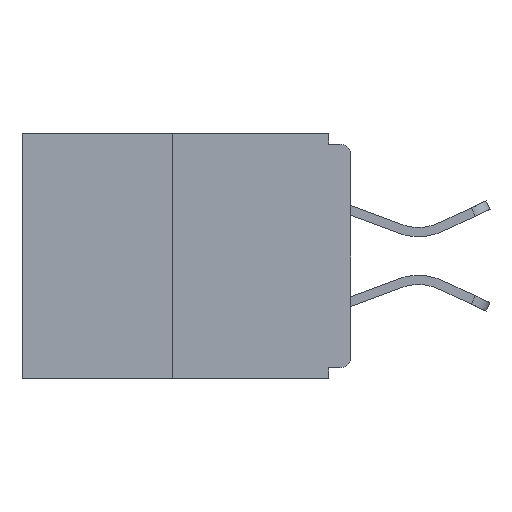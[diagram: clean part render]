
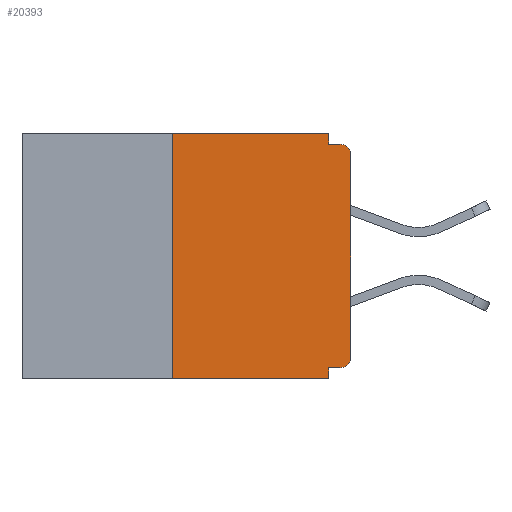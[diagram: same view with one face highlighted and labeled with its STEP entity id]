
A CAD part, left-side view. The second image highlights one B-rep face of the part: STEP entity #20393.
In plain terms, the highlighted planar face has unit normal (-1, 0, 0).
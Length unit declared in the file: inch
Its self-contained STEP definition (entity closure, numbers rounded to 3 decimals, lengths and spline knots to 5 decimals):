
#811 = DIRECTION ( 'NONE',  ( 0., -1., 0. ) ) ;
#1473 = CARTESIAN_POINT ( 'NONE',  ( 0., 0.031, 0. ) ) ;
#1618 = VECTOR ( 'NONE', #811, 39.37008 ) ;
#1887 = VERTEX_POINT ( 'NONE', #28854 ) ;
#2306 = CARTESIAN_POINT ( 'NONE',  ( 0., 0.015, -0.015 ) ) ;
#2321 = VERTEX_POINT ( 'NONE', #1473 ) ;
#2989 = DIRECTION ( 'NONE',  ( 1., 0., 0. ) ) ;
#3128 = CARTESIAN_POINT ( 'NONE',  ( 0., 0.015, -0.328 ) ) ;
#3155 = DIRECTION ( 'NONE',  ( 0., -1., 0. ) ) ;
#3368 = LINE ( 'NONE', #21479, #1618 ) ;
#3377 = VERTEX_POINT ( 'NONE', #6656 ) ;
#3804 = CARTESIAN_POINT ( 'NONE',  ( 0., 0.25, 0. ) ) ;
#4388 = AXIS2_PLACEMENT_3D ( 'NONE', #17617, #29236, #29541 ) ;
#4418 = CARTESIAN_POINT ( 'NONE',  ( 0., 0., -0.313 ) ) ;
#4719 = ORIENTED_EDGE ( 'NONE', *, *, #23878, .F. ) ;
#4732 = VERTEX_POINT ( 'NONE', #3804 ) ;
#4808 = VECTOR ( 'NONE', #23315, 39.37008 ) ;
#5930 = VERTEX_POINT ( 'NONE', #7351 ) ;
#6019 = LINE ( 'NONE', #22008, #26554 ) ;
#6042 = ORIENTED_EDGE ( 'NONE', *, *, #11639, .F. ) ;
#6083 = CARTESIAN_POINT ( 'NONE',  ( 0., 0.031, 0. ) ) ;
#6374 = LINE ( 'NONE', #18257, #24286 ) ;
#6656 = CARTESIAN_POINT ( 'NONE',  ( 0., 0.031, -0.015 ) ) ;
#7351 = CARTESIAN_POINT ( 'NONE',  ( 0., 0.031, -0.328 ) ) ;
#8089 = PLANE ( 'NONE',  #16899 ) ;
#9112 = EDGE_CURVE ( 'NONE', #13773, #11998, #25568, .T. ) ;
#9196 = CARTESIAN_POINT ( 'NONE',  ( 0., 0., -0.328 ) ) ;
#10501 = EDGE_CURVE ( 'NONE', #18077, #13773, #27045, .T. ) ;
#11170 = EDGE_LOOP ( 'NONE', ( #15086, #4719, #16507, #25999, #6042, #23730, #26352, #15635, #24366, #24740 ) ) ;
#11278 = CARTESIAN_POINT ( 'NONE',  ( 0., 0.015, -0.03 ) ) ;
#11639 = EDGE_CURVE ( 'NONE', #18077, #5930, #27781, .T. ) ;
#11921 = DIRECTION ( 'NONE',  ( 0., 1., 0. ) ) ;
#11998 = VERTEX_POINT ( 'NONE', #24683 ) ;
#12180 = DIRECTION ( 'NONE',  ( 0., 0., -1. ) ) ;
#13393 = CIRCLE ( 'NONE', #18190, 0.015 ) ;
#13605 = DIRECTION ( 'NONE',  ( 0., 0., 1. ) ) ;
#13750 = VERTEX_POINT ( 'NONE', #2306 ) ;
#13773 = VERTEX_POINT ( 'NONE', #4418 ) ;
#14049 = EDGE_CURVE ( 'NONE', #11998, #13750, #13393, .T. ) ;
#14098 = CARTESIAN_POINT ( 'NONE',  ( 0., 0., 0. ) ) ;
#14428 = FACE_OUTER_BOUND ( 'NONE', #11170, .T. ) ;
#15086 = ORIENTED_EDGE ( 'NONE', *, *, #26963, .F. ) ;
#15635 = ORIENTED_EDGE ( 'NONE', *, *, #14049, .T. ) ;
#15809 = CARTESIAN_POINT ( 'NONE',  ( 0., 0.031, -0.343 ) ) ;
#16507 = ORIENTED_EDGE ( 'NONE', *, *, #20335, .T. ) ;
#16899 = AXIS2_PLACEMENT_3D ( 'NONE', #23639, #2989, #12180 ) ;
#17395 = DIRECTION ( 'NONE',  ( 0., 0., -1. ) ) ;
#17617 = CARTESIAN_POINT ( 'NONE',  ( 0., 0.015, -0.313 ) ) ;
#18077 = VERTEX_POINT ( 'NONE', #3128 ) ;
#18190 = AXIS2_PLACEMENT_3D ( 'NONE', #11278, #20498, #29687 ) ;
#18257 = CARTESIAN_POINT ( 'NONE',  ( 0., 0.25, 0. ) ) ;
#20335 = EDGE_CURVE ( 'NONE', #20956, #1887, #26502, .T. ) ;
#20393 = ADVANCED_FACE ( 'NONE', ( #14428 ), #8089, .F. ) ;
#20498 = DIRECTION ( 'NONE',  ( -1., 0., 0. ) ) ;
#20956 = VERTEX_POINT ( 'NONE', #24491 ) ;
#21285 = VECTOR ( 'NONE', #29397, 39.37008 ) ;
#21406 = EDGE_CURVE ( 'NONE', #5930, #1887, #26986, .T. ) ;
#21479 = CARTESIAN_POINT ( 'NONE',  ( 0., 0., -0.015 ) ) ;
#22008 = CARTESIAN_POINT ( 'NONE',  ( 0., 0.46, 0. ) ) ;
#22554 = EDGE_CURVE ( 'NONE', #3377, #13750, #3368, .T. ) ;
#23315 = DIRECTION ( 'NONE',  ( 0., 0., 1. ) ) ;
#23639 = CARTESIAN_POINT ( 'NONE',  ( 0., 0.46, 0. ) ) ;
#23730 = ORIENTED_EDGE ( 'NONE', *, *, #10501, .T. ) ;
#23813 = CARTESIAN_POINT ( 'NONE',  ( 0., 0.46, -0.343 ) ) ;
#23878 = EDGE_CURVE ( 'NONE', #20956, #4732, #6374, .T. ) ;
#24286 = VECTOR ( 'NONE', #13605, 39.37008 ) ;
#24366 = ORIENTED_EDGE ( 'NONE', *, *, #22554, .F. ) ;
#24491 = CARTESIAN_POINT ( 'NONE',  ( 0., 0.25, -0.343 ) ) ;
#24683 = CARTESIAN_POINT ( 'NONE',  ( 0., 0., -0.03 ) ) ;
#24740 = ORIENTED_EDGE ( 'NONE', *, *, #26066, .F. ) ;
#25085 = VECTOR ( 'NONE', #3155, 39.37008 ) ;
#25568 = LINE ( 'NONE', #14098, #4808 ) ;
#25999 = ORIENTED_EDGE ( 'NONE', *, *, #21406, .F. ) ;
#26066 = EDGE_CURVE ( 'NONE', #2321, #3377, #26331, .T. ) ;
#26331 = LINE ( 'NONE', #6083, #27448 ) ;
#26352 = ORIENTED_EDGE ( 'NONE', *, *, #9112, .T. ) ;
#26502 = LINE ( 'NONE', #23813, #25085 ) ;
#26536 = DIRECTION ( 'NONE',  ( 0., -1., 0. ) ) ;
#26554 = VECTOR ( 'NONE', #26536, 39.37008 ) ;
#26963 = EDGE_CURVE ( 'NONE', #4732, #2321, #6019, .T. ) ;
#26986 = LINE ( 'NONE', #15809, #21285 ) ;
#27045 = CIRCLE ( 'NONE', #4388, 0.015 ) ;
#27448 = VECTOR ( 'NONE', #17395, 39.37008 ) ;
#27781 = LINE ( 'NONE', #9196, #29509 ) ;
#28854 = CARTESIAN_POINT ( 'NONE',  ( 0., 0.031, -0.343 ) ) ;
#29236 = DIRECTION ( 'NONE',  ( -1., 0., 0. ) ) ;
#29397 = DIRECTION ( 'NONE',  ( 0., 0., -1. ) ) ;
#29509 = VECTOR ( 'NONE', #11921, 39.37008 ) ;
#29541 = DIRECTION ( 'NONE',  ( 0., 0., -1. ) ) ;
#29687 = DIRECTION ( 'NONE',  ( 0., 0., -1. ) ) ;
